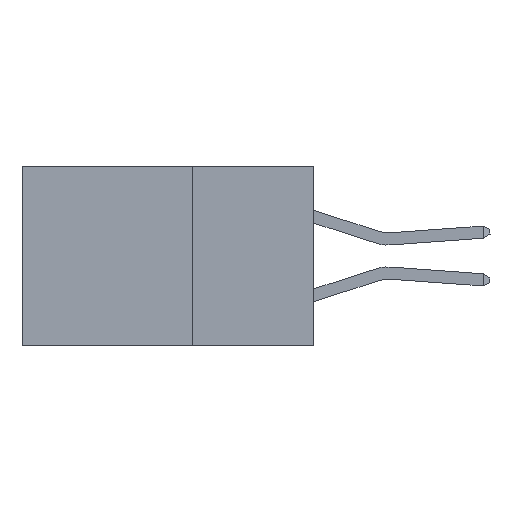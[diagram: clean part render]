
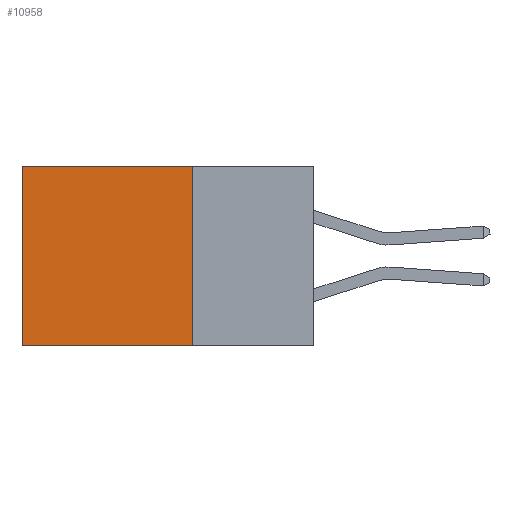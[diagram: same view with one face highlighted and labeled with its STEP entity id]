
A CAD part, left-side view. The second image highlights one B-rep face of the part: STEP entity #10958.
In plain terms, the highlighted planar face has unit normal (-1, 0, 0).
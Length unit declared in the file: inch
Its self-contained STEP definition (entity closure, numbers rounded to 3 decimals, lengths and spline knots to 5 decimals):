
#41 = EDGE_CURVE ( 'NONE', #8488, #1462, #6073, .T. ) ;
#159 = EDGE_CURVE ( 'NONE', #3611, #3646, #9474, .T. ) ;
#165 = DIRECTION ( 'NONE',  ( 1., 0., 0. ) ) ;
#442 = VECTOR ( 'NONE', #2987, 39.37008 ) ;
#1054 = DIRECTION ( 'NONE',  ( 0., 1., 0. ) ) ;
#1214 = VECTOR ( 'NONE', #9386, 39.37008 ) ;
#1363 = ORIENTED_EDGE ( 'NONE', *, *, #41, .T. ) ;
#1462 = VERTEX_POINT ( 'NONE', #7494 ) ;
#1697 = ORIENTED_EDGE ( 'NONE', *, *, #9401, .T. ) ;
#1804 = CARTESIAN_POINT ( 'NONE',  ( 0.2875, 0.6, -0.37 ) ) ;
#1968 = CARTESIAN_POINT ( 'NONE',  ( 0.2875, 0.25, -0.37 ) ) ;
#2987 = DIRECTION ( 'NONE',  ( 0., 0., -1. ) ) ;
#3326 = DIRECTION ( 'NONE',  ( 0., 1., 0. ) ) ;
#3611 = VERTEX_POINT ( 'NONE', #1968 ) ;
#3646 = VERTEX_POINT ( 'NONE', #1804 ) ;
#3690 = DIRECTION ( 'NONE',  ( 0., 0., -1. ) ) ;
#4495 = CARTESIAN_POINT ( 'NONE',  ( 0.2875, 0.25, 0. ) ) ;
#4714 = CARTESIAN_POINT ( 'NONE',  ( 0.2875, 0.25, 0. ) ) ;
#5112 = CARTESIAN_POINT ( 'NONE',  ( 0.2875, 0.25, 0. ) ) ;
#5880 = CARTESIAN_POINT ( 'NONE',  ( 0.2875, 0.6, 0. ) ) ;
#6073 = LINE ( 'NONE', #11379, #10485 ) ;
#6566 = EDGE_CURVE ( 'NONE', #8488, #3611, #10859, .T. ) ;
#6829 = AXIS2_PLACEMENT_3D ( 'NONE', #4495, #165, #3690 ) ;
#7494 = CARTESIAN_POINT ( 'NONE',  ( 0.2875, 0.6, 0. ) ) ;
#7942 = FACE_OUTER_BOUND ( 'NONE', #9429, .T. ) ;
#8488 = VERTEX_POINT ( 'NONE', #5112 ) ;
#8857 = PLANE ( 'NONE',  #6829 ) ;
#8946 = CARTESIAN_POINT ( 'NONE',  ( 0.2875, 0.25, -0.37 ) ) ;
#9386 = DIRECTION ( 'NONE',  ( 0., 0., -1. ) ) ;
#9401 = EDGE_CURVE ( 'NONE', #1462, #3646, #10236, .T. ) ;
#9416 = VECTOR ( 'NONE', #1054, 39.37008 ) ;
#9429 = EDGE_LOOP ( 'NONE', ( #1697, #11025, #10513, #1363 ) ) ;
#9474 = LINE ( 'NONE', #8946, #9416 ) ;
#10236 = LINE ( 'NONE', #5880, #1214 ) ;
#10485 = VECTOR ( 'NONE', #3326, 39.37008 ) ;
#10513 = ORIENTED_EDGE ( 'NONE', *, *, #6566, .F. ) ;
#10859 = LINE ( 'NONE', #4714, #442 ) ;
#10958 = ADVANCED_FACE ( 'NONE', ( #7942 ), #8857, .F. ) ;
#11025 = ORIENTED_EDGE ( 'NONE', *, *, #159, .F. ) ;
#11379 = CARTESIAN_POINT ( 'NONE',  ( 0.2875, 0.25, 0. ) ) ;
